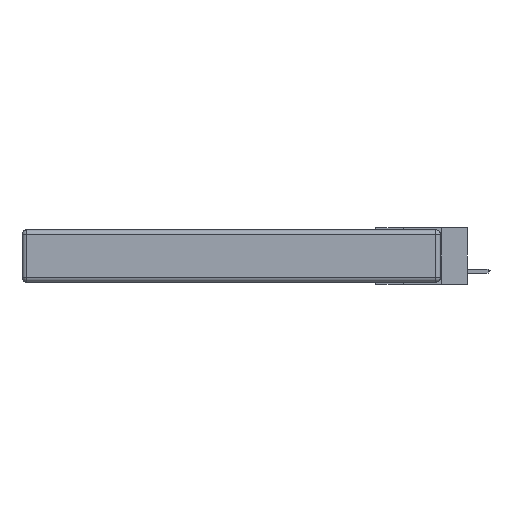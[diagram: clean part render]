
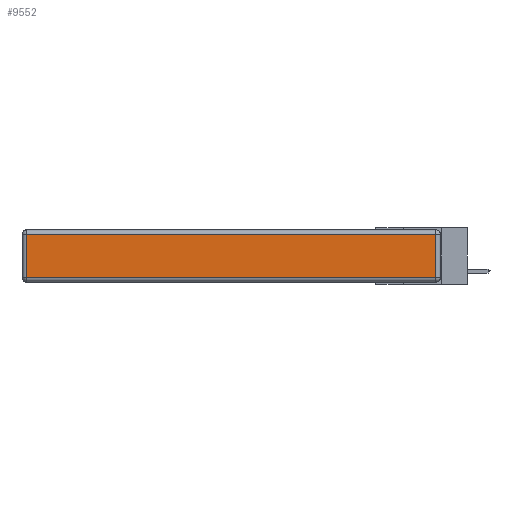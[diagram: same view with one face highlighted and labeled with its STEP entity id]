
A CAD part, left-side view. The second image highlights one B-rep face of the part: STEP entity #9552.
In plain terms, the highlighted planar face has unit normal (-1, 0, 0).
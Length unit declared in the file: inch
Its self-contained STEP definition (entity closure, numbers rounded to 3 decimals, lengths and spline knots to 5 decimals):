
#456 = DIRECTION ( 'NONE',  ( 0., -1., 0. ) ) ;
#477 = DIRECTION ( 'NONE',  ( 0., 1., 0. ) ) ;
#1574 = PLANE ( 'NONE',  #26336 ) ;
#3950 = DIRECTION ( 'NONE',  ( 0., 0., 1. ) ) ;
#6451 = VERTEX_POINT ( 'NONE', #16627 ) ;
#7222 = LINE ( 'NONE', #23656, #11655 ) ;
#8529 = CARTESIAN_POINT ( 'NONE',  ( 0., 2.72, -0.343 ) ) ;
#8976 = EDGE_CURVE ( 'NONE', #26686, #6451, #30664, .T. ) ;
#9552 = ADVANCED_FACE ( 'NONE', ( #15311 ), #1574, .T. ) ;
#9946 = VECTOR ( 'NONE', #477, 39.37008 ) ;
#9969 = ORIENTED_EDGE ( 'NONE', *, *, #10692, .T. ) ;
#10692 = EDGE_CURVE ( 'NONE', #26871, #26686, #30625, .T. ) ;
#11104 = DIRECTION ( 'NONE',  ( 0., 0., -1. ) ) ;
#11655 = VECTOR ( 'NONE', #456, 39.37008 ) ;
#12909 = VERTEX_POINT ( 'NONE', #13027 ) ;
#13027 = CARTESIAN_POINT ( 'NONE',  ( 0., 0.03, -0.313 ) ) ;
#15311 = FACE_OUTER_BOUND ( 'NONE', #28256, .T. ) ;
#16627 = CARTESIAN_POINT ( 'NONE',  ( 0., 2.72, -0.313 ) ) ;
#16673 = LINE ( 'NONE', #21507, #21830 ) ;
#16850 = DIRECTION ( 'NONE',  ( -1., 0., 0. ) ) ;
#18369 = CARTESIAN_POINT ( 'NONE',  ( 0., 2.72, -0.03 ) ) ;
#18827 = CARTESIAN_POINT ( 'NONE',  ( 0., 0.03, -0.03 ) ) ;
#19032 = ORIENTED_EDGE ( 'NONE', *, *, #8976, .T. ) ;
#20018 = ORIENTED_EDGE ( 'NONE', *, *, #28374, .T. ) ;
#21507 = CARTESIAN_POINT ( 'NONE',  ( 0., 0.03, -0.343 ) ) ;
#21830 = VECTOR ( 'NONE', #24414, 39.37008 ) ;
#22880 = EDGE_CURVE ( 'NONE', #6451, #12909, #7222, .T. ) ;
#22979 = VECTOR ( 'NONE', #11104, 39.37008 ) ;
#23656 = CARTESIAN_POINT ( 'NONE',  ( 0., 0., -0.313 ) ) ;
#24414 = DIRECTION ( 'NONE',  ( 0., 0., 1. ) ) ;
#26336 = AXIS2_PLACEMENT_3D ( 'NONE', #32392, #16850, #3950 ) ;
#26686 = VERTEX_POINT ( 'NONE', #18369 ) ;
#26871 = VERTEX_POINT ( 'NONE', #18827 ) ;
#28256 = EDGE_LOOP ( 'NONE', ( #30298, #20018, #9969, #19032 ) ) ;
#28374 = EDGE_CURVE ( 'NONE', #12909, #26871, #16673, .T. ) ;
#30298 = ORIENTED_EDGE ( 'NONE', *, *, #22880, .T. ) ;
#30625 = LINE ( 'NONE', #31264, #9946 ) ;
#30664 = LINE ( 'NONE', #8529, #22979 ) ;
#31264 = CARTESIAN_POINT ( 'NONE',  ( 0., 2.75, -0.03 ) ) ;
#32392 = CARTESIAN_POINT ( 'NONE',  ( 0., 0., -0.343 ) ) ;
